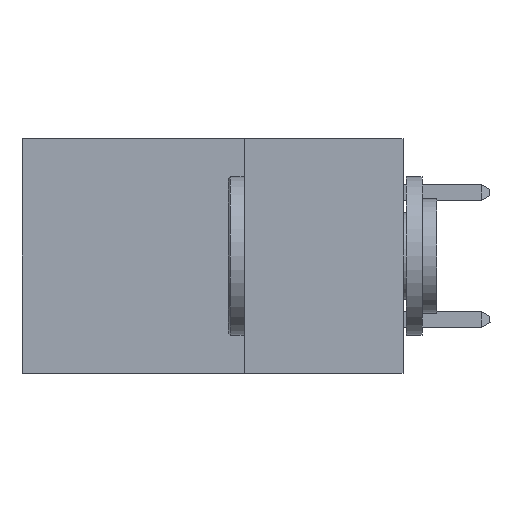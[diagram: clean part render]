
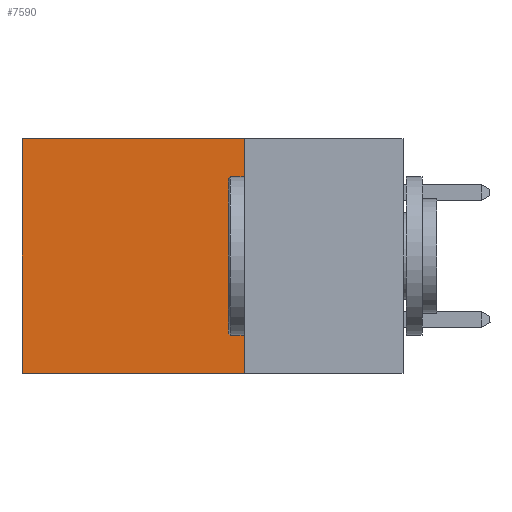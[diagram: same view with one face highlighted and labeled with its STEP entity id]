
A CAD part, left-side view. The second image highlights one B-rep face of the part: STEP entity #7590.
In plain terms, the highlighted planar face has unit normal (-1, 0, 0).
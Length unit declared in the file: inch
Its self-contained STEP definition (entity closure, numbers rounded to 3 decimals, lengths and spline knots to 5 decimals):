
#371 = LINE ( 'NONE', #17899, #2470 ) ;
#885 = VERTEX_POINT ( 'NONE', #21752 ) ;
#1125 = VECTOR ( 'NONE', #7228, 39.37008 ) ;
#1270 = LINE ( 'NONE', #1334, #23934 ) ;
#1334 = CARTESIAN_POINT ( 'NONE',  ( 0.2875, 0.25, 0. ) ) ;
#1713 = DIRECTION ( 'NONE',  ( 0., 0., -1. ) ) ;
#2224 = AXIS2_PLACEMENT_3D ( 'NONE', #16574, #14454, #27627 ) ;
#2470 = VECTOR ( 'NONE', #11458, 39.37008 ) ;
#3409 = ORIENTED_EDGE ( 'NONE', *, *, #21056, .T. ) ;
#4540 = CARTESIAN_POINT ( 'NONE',  ( 0.2875, 0.6, -0.37 ) ) ;
#4689 = ORIENTED_EDGE ( 'NONE', *, *, #25309, .F. ) ;
#7084 = ORIENTED_EDGE ( 'NONE', *, *, #11673, .T. ) ;
#7228 = DIRECTION ( 'NONE',  ( 0., 0., -1. ) ) ;
#7590 = ADVANCED_FACE ( 'NONE', ( #9081 ), #16298, .F. ) ;
#9081 = FACE_OUTER_BOUND ( 'NONE', #17013, .T. ) ;
#10498 = VECTOR ( 'NONE', #24159, 39.37008 ) ;
#11458 = DIRECTION ( 'NONE',  ( 0., 1., 0. ) ) ;
#11673 = EDGE_CURVE ( 'NONE', #16964, #23230, #19641, .T. ) ;
#11899 = VERTEX_POINT ( 'NONE', #22746 ) ;
#12453 = EDGE_CURVE ( 'NONE', #11899, #23230, #371, .T. ) ;
#14454 = DIRECTION ( 'NONE',  ( 1., 0., 0. ) ) ;
#15278 = LINE ( 'NONE', #15399, #10498 ) ;
#15399 = CARTESIAN_POINT ( 'NONE',  ( 0.2875, 0.25, 0. ) ) ;
#16298 = PLANE ( 'NONE',  #2224 ) ;
#16574 = CARTESIAN_POINT ( 'NONE',  ( 0.2875, 0.25, 0. ) ) ;
#16964 = VERTEX_POINT ( 'NONE', #24150 ) ;
#17013 = EDGE_LOOP ( 'NONE', ( #7084, #24057, #4689, #3409 ) ) ;
#17842 = CARTESIAN_POINT ( 'NONE',  ( 0.2875, 0.6, 0. ) ) ;
#17899 = CARTESIAN_POINT ( 'NONE',  ( 0.2875, 0.25, -0.37 ) ) ;
#19641 = LINE ( 'NONE', #17842, #1125 ) ;
#21056 = EDGE_CURVE ( 'NONE', #885, #16964, #15278, .T. ) ;
#21752 = CARTESIAN_POINT ( 'NONE',  ( 0.2875, 0.25, 0. ) ) ;
#22746 = CARTESIAN_POINT ( 'NONE',  ( 0.2875, 0.25, -0.37 ) ) ;
#23230 = VERTEX_POINT ( 'NONE', #4540 ) ;
#23934 = VECTOR ( 'NONE', #1713, 39.37008 ) ;
#24057 = ORIENTED_EDGE ( 'NONE', *, *, #12453, .F. ) ;
#24150 = CARTESIAN_POINT ( 'NONE',  ( 0.2875, 0.6, 0. ) ) ;
#24159 = DIRECTION ( 'NONE',  ( 0., 1., 0. ) ) ;
#25309 = EDGE_CURVE ( 'NONE', #885, #11899, #1270, .T. ) ;
#27627 = DIRECTION ( 'NONE',  ( 0., 0., -1. ) ) ;
